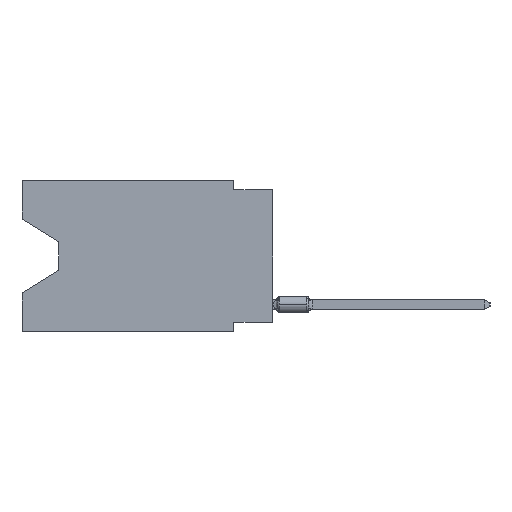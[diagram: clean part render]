
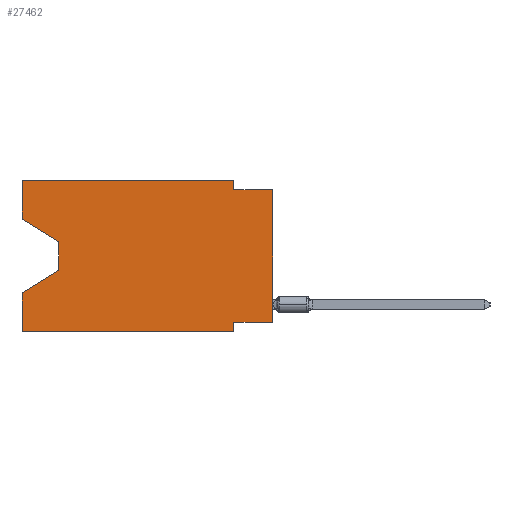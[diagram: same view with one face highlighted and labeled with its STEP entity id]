
A CAD part, left-side view. The second image highlights one B-rep face of the part: STEP entity #27462.
In plain terms, the highlighted planar face has unit normal (-1, 0, 0).
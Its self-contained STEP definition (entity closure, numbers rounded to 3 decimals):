
#8 = CARTESIAN_POINT ( 'NONE',  ( 0., 13.97, -5.893 ) ) ;
#222 = VERTEX_POINT ( 'NONE', #35640 ) ;
#552 = ORIENTED_EDGE ( 'NONE', *, *, #10451, .T. ) ;
#962 = LINE ( 'NONE', #30989, #20040 ) ;
#1417 = CARTESIAN_POINT ( 'NONE',  ( 0., 16.383, -9.906 ) ) ;
#1554 = LINE ( 'NONE', #33051, #9296 ) ;
#2682 = VERTEX_POINT ( 'NONE', #25823 ) ;
#2893 = VERTEX_POINT ( 'NONE', #31608 ) ;
#3410 = CARTESIAN_POINT ( 'NONE',  ( 0., 0., -0.635 ) ) ;
#3608 = CARTESIAN_POINT ( 'NONE',  ( 0., 16.383, -9.906 ) ) ;
#3785 = ORIENTED_EDGE ( 'NONE', *, *, #15551, .T. ) ;
#4287 = VERTEX_POINT ( 'NONE', #11371 ) ;
#4406 = LINE ( 'NONE', #24504, #24302 ) ;
#4463 = DIRECTION ( 'NONE',  ( 0., 0., -1. ) ) ;
#4502 = VERTEX_POINT ( 'NONE', #33881 ) ;
#5010 = VECTOR ( 'NONE', #15498, 1000. ) ;
#5046 = ORIENTED_EDGE ( 'NONE', *, *, #20680, .T. ) ;
#6064 = DIRECTION ( 'NONE',  ( 0., -1., 0. ) ) ;
#6666 = VERTEX_POINT ( 'NONE', #3608 ) ;
#7475 = CARTESIAN_POINT ( 'NONE',  ( 0., 16.383, 0. ) ) ;
#7619 = EDGE_LOOP ( 'NONE', ( #5046, #552, #18636, #31463, #11496, #20571, #36400, #3785, #33592, #20001, #32093, #22141 ) ) ;
#7800 = EDGE_CURVE ( 'NONE', #2893, #16982, #1554, .T. ) ;
#8668 = CARTESIAN_POINT ( 'NONE',  ( 0., 16.383, -7.36 ) ) ;
#8776 = VECTOR ( 'NONE', #15166, 1000. ) ;
#8881 = AXIS2_PLACEMENT_3D ( 'NONE', #7475, #30248, #4463 ) ;
#9296 = VECTOR ( 'NONE', #27523, 1000. ) ;
#9430 = LINE ( 'NONE', #29711, #5010 ) ;
#9645 = VERTEX_POINT ( 'NONE', #10092 ) ;
#9672 = DIRECTION ( 'NONE',  ( 0., 0.855, -0.519 ) ) ;
#10092 = CARTESIAN_POINT ( 'NONE',  ( 0., 0., -9.271 ) ) ;
#10451 = EDGE_CURVE ( 'NONE', #33480, #4502, #962, .T. ) ;
#10578 = EDGE_CURVE ( 'NONE', #9645, #16911, #17534, .T. ) ;
#10666 = EDGE_CURVE ( 'NONE', #4287, #222, #26461, .T. ) ;
#10873 = DIRECTION ( 'NONE',  ( 0., -1., 0. ) ) ;
#11371 = CARTESIAN_POINT ( 'NONE',  ( 0., 2.54, 0. ) ) ;
#11496 = ORIENTED_EDGE ( 'NONE', *, *, #25277, .T. ) ;
#12692 = LINE ( 'NONE', #23706, #8776 ) ;
#12930 = DIRECTION ( 'NONE',  ( 0., 0., 1. ) ) ;
#13375 = EDGE_CURVE ( 'NONE', #222, #2682, #14772, .T. ) ;
#13750 = DIRECTION ( 'NONE',  ( 0., 1., 0. ) ) ;
#14139 = VECTOR ( 'NONE', #9672, 1000. ) ;
#14631 = VERTEX_POINT ( 'NONE', #18894 ) ;
#14772 = LINE ( 'NONE', #3410, #35739 ) ;
#14965 = CARTESIAN_POINT ( 'NONE',  ( 0., 2.54, -9.271 ) ) ;
#15166 = DIRECTION ( 'NONE',  ( 0., 0., 1. ) ) ;
#15498 = DIRECTION ( 'NONE',  ( 0., -1., 0. ) ) ;
#15550 = DIRECTION ( 'NONE',  ( 0., 0., -1. ) ) ;
#15551 = EDGE_CURVE ( 'NONE', #9645, #2682, #4406, .T. ) ;
#16911 = VERTEX_POINT ( 'NONE', #14965 ) ;
#16982 = VERTEX_POINT ( 'NONE', #21910 ) ;
#17534 = LINE ( 'NONE', #31378, #27880 ) ;
#17619 = VECTOR ( 'NONE', #29109, 1000. ) ;
#18636 = ORIENTED_EDGE ( 'NONE', *, *, #34760, .T. ) ;
#18864 = PLANE ( 'NONE',  #8881 ) ;
#18894 = CARTESIAN_POINT ( 'NONE',  ( 0., 2.54, -9.906 ) ) ;
#20001 = ORIENTED_EDGE ( 'NONE', *, *, #10666, .F. ) ;
#20040 = VECTOR ( 'NONE', #15550, 1000. ) ;
#20433 = CARTESIAN_POINT ( 'NONE',  ( 0., 16.383, -2.546 ) ) ;
#20571 = ORIENTED_EDGE ( 'NONE', *, *, #24853, .F. ) ;
#20609 = DIRECTION ( 'NONE',  ( 0., -0.855, -0.519 ) ) ;
#20680 = EDGE_CURVE ( 'NONE', #2893, #33480, #32187, .T. ) ;
#21910 = CARTESIAN_POINT ( 'NONE',  ( 0., 16.383, 0. ) ) ;
#22141 = ORIENTED_EDGE ( 'NONE', *, *, #7800, .F. ) ;
#22279 = DIRECTION ( 'NONE',  ( 0., 0., -1. ) ) ;
#22863 = VECTOR ( 'NONE', #22279, 1000. ) ;
#23706 = CARTESIAN_POINT ( 'NONE',  ( 0., 16.383, 0. ) ) ;
#23892 = CARTESIAN_POINT ( 'NONE',  ( 0., 13.97, -4.013 ) ) ;
#24302 = VECTOR ( 'NONE', #12930, 1000. ) ;
#24504 = CARTESIAN_POINT ( 'NONE',  ( 0., 0., 0. ) ) ;
#24853 = EDGE_CURVE ( 'NONE', #16911, #14631, #36861, .T. ) ;
#25277 = EDGE_CURVE ( 'NONE', #6666, #14631, #27388, .T. ) ;
#25823 = CARTESIAN_POINT ( 'NONE',  ( 0., 0., -0.635 ) ) ;
#25961 = LINE ( 'NONE', #8, #14139 ) ;
#26461 = LINE ( 'NONE', #34994, #17619 ) ;
#26470 = EDGE_CURVE ( 'NONE', #6666, #33774, #12692, .T. ) ;
#27388 = LINE ( 'NONE', #1417, #27723 ) ;
#27462 = ADVANCED_FACE ( 'NONE', ( #32921 ), #18864, .F. ) ;
#27523 = DIRECTION ( 'NONE',  ( 0., 0., 1. ) ) ;
#27723 = VECTOR ( 'NONE', #10873, 1000. ) ;
#27880 = VECTOR ( 'NONE', #13750, 1000. ) ;
#28181 = VECTOR ( 'NONE', #20609, 1000. ) ;
#29109 = DIRECTION ( 'NONE',  ( 0., 0., -1. ) ) ;
#29711 = CARTESIAN_POINT ( 'NONE',  ( 0., 16.383, 0. ) ) ;
#30248 = DIRECTION ( 'NONE',  ( 1., 0., 0. ) ) ;
#30989 = CARTESIAN_POINT ( 'NONE',  ( 0., 13.97, -4.013 ) ) ;
#31378 = CARTESIAN_POINT ( 'NONE',  ( 0., 0., -9.271 ) ) ;
#31463 = ORIENTED_EDGE ( 'NONE', *, *, #26470, .F. ) ;
#31608 = CARTESIAN_POINT ( 'NONE',  ( 0., 16.383, -2.546 ) ) ;
#32093 = ORIENTED_EDGE ( 'NONE', *, *, #33889, .F. ) ;
#32187 = LINE ( 'NONE', #20433, #28181 ) ;
#32921 = FACE_OUTER_BOUND ( 'NONE', #7619, .T. ) ;
#33051 = CARTESIAN_POINT ( 'NONE',  ( 0., 16.383, 0. ) ) ;
#33480 = VERTEX_POINT ( 'NONE', #23892 ) ;
#33481 = CARTESIAN_POINT ( 'NONE',  ( 0., 2.54, -9.906 ) ) ;
#33592 = ORIENTED_EDGE ( 'NONE', *, *, #13375, .F. ) ;
#33774 = VERTEX_POINT ( 'NONE', #8668 ) ;
#33881 = CARTESIAN_POINT ( 'NONE',  ( 0., 13.97, -5.893 ) ) ;
#33889 = EDGE_CURVE ( 'NONE', #16982, #4287, #9430, .T. ) ;
#34760 = EDGE_CURVE ( 'NONE', #4502, #33774, #25961, .T. ) ;
#34994 = CARTESIAN_POINT ( 'NONE',  ( 0., 2.54, 0. ) ) ;
#35640 = CARTESIAN_POINT ( 'NONE',  ( 0., 2.54, -0.635 ) ) ;
#35739 = VECTOR ( 'NONE', #6064, 1000. ) ;
#36400 = ORIENTED_EDGE ( 'NONE', *, *, #10578, .F. ) ;
#36861 = LINE ( 'NONE', #33481, #22863 ) ;
